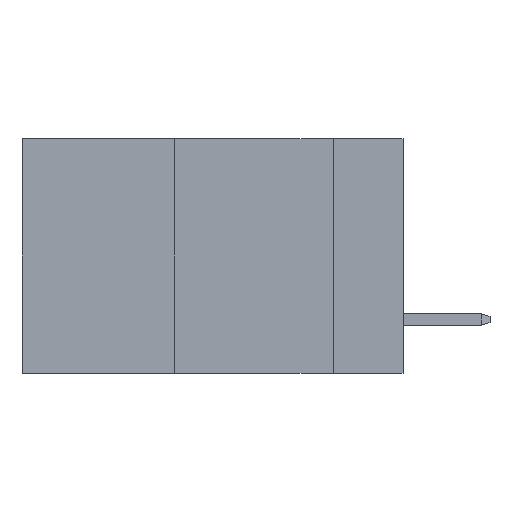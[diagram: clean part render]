
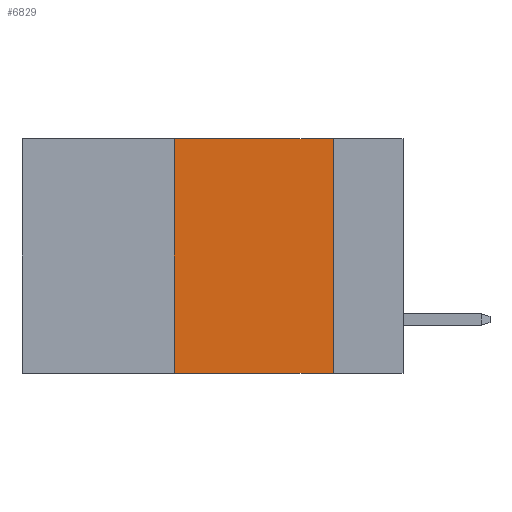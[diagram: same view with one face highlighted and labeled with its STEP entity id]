
A CAD part, left-side view. The second image highlights one B-rep face of the part: STEP entity #6829.
In plain terms, the highlighted planar face has unit normal (-1, 0, 0).
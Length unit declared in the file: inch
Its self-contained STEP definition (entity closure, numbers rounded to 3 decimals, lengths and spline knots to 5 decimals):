
#180 = CARTESIAN_POINT ( 'NONE',  ( 0., 0.11, 0. ) ) ;
#305 = LINE ( 'NONE', #4782, #8745 ) ;
#386 = VECTOR ( 'NONE', #2437, 39.37008 ) ;
#712 = PLANE ( 'NONE',  #3177 ) ;
#868 = VERTEX_POINT ( 'NONE', #9267 ) ;
#1426 = FACE_OUTER_BOUND ( 'NONE', #2900, .T. ) ;
#1568 = LINE ( 'NONE', #7564, #8209 ) ;
#1715 = DIRECTION ( 'NONE',  ( 0., 0., 1. ) ) ;
#2259 = EDGE_CURVE ( 'NONE', #868, #8181, #1568, .T. ) ;
#2437 = DIRECTION ( 'NONE',  ( 0., -1., 0. ) ) ;
#2797 = DIRECTION ( 'NONE',  ( 1., 0., 0. ) ) ;
#2900 = EDGE_LOOP ( 'NONE', ( #3758, #3645, #4803, #6061 ) ) ;
#2946 = DIRECTION ( 'NONE',  ( 0., 0., -1. ) ) ;
#3177 = AXIS2_PLACEMENT_3D ( 'NONE', #8853, #2797, #2946 ) ;
#3627 = CARTESIAN_POINT ( 'NONE',  ( 0., 0.11, -0.37 ) ) ;
#3645 = ORIENTED_EDGE ( 'NONE', *, *, #2259, .F. ) ;
#3698 = DIRECTION ( 'NONE',  ( 0., -1., 0. ) ) ;
#3758 = ORIENTED_EDGE ( 'NONE', *, *, #8187, .F. ) ;
#3965 = CARTESIAN_POINT ( 'NONE',  ( 0., 0.11, 0. ) ) ;
#4138 = VERTEX_POINT ( 'NONE', #3627 ) ;
#4782 = CARTESIAN_POINT ( 'NONE',  ( 0., 0.36, 0. ) ) ;
#4803 = ORIENTED_EDGE ( 'NONE', *, *, #7406, .F. ) ;
#4806 = VERTEX_POINT ( 'NONE', #4996 ) ;
#4996 = CARTESIAN_POINT ( 'NONE',  ( 0., 0.36, -0.37 ) ) ;
#6061 = ORIENTED_EDGE ( 'NONE', *, *, #9060, .T. ) ;
#6200 = DIRECTION ( 'NONE',  ( 0., 0., -1. ) ) ;
#6765 = LINE ( 'NONE', #8205, #386 ) ;
#6829 = ADVANCED_FACE ( 'NONE', ( #1426 ), #712, .F. ) ;
#7223 = VECTOR ( 'NONE', #6200, 39.37008 ) ;
#7406 = EDGE_CURVE ( 'NONE', #4806, #868, #305, .T. ) ;
#7564 = CARTESIAN_POINT ( 'NONE',  ( 0., 0.6, 0. ) ) ;
#8181 = VERTEX_POINT ( 'NONE', #180 ) ;
#8187 = EDGE_CURVE ( 'NONE', #8181, #4138, #8997, .T. ) ;
#8205 = CARTESIAN_POINT ( 'NONE',  ( 0., 0.6, -0.37 ) ) ;
#8209 = VECTOR ( 'NONE', #3698, 39.37008 ) ;
#8745 = VECTOR ( 'NONE', #1715, 39.37008 ) ;
#8853 = CARTESIAN_POINT ( 'NONE',  ( 0., 0.6, 0. ) ) ;
#8997 = LINE ( 'NONE', #3965, #7223 ) ;
#9060 = EDGE_CURVE ( 'NONE', #4806, #4138, #6765, .T. ) ;
#9267 = CARTESIAN_POINT ( 'NONE',  ( 0., 0.36, 0. ) ) ;
